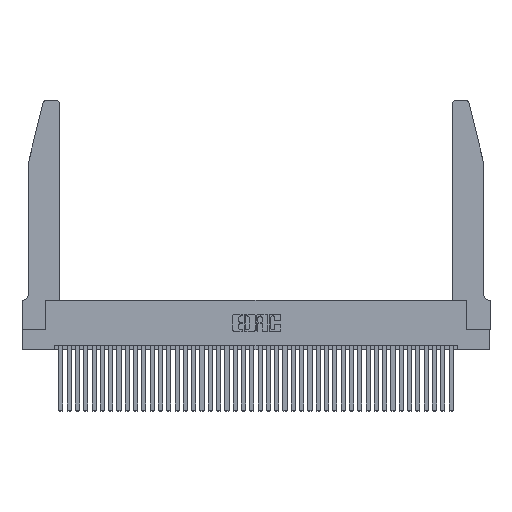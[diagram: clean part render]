
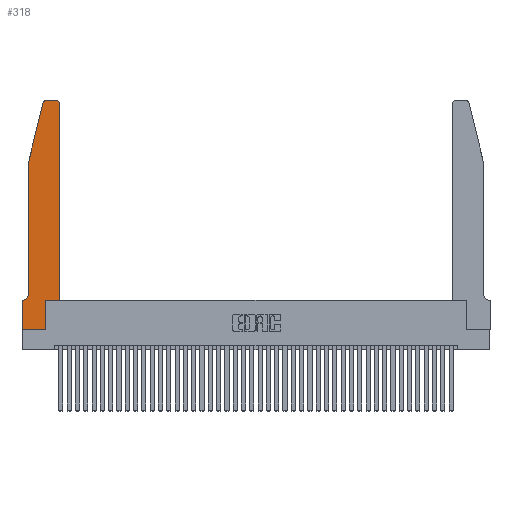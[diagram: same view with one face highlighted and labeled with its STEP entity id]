
A CAD part, top view. The second image highlights one B-rep face of the part: STEP entity #318.
In plain terms, the highlighted planar face has unit normal (0, 0, 1).
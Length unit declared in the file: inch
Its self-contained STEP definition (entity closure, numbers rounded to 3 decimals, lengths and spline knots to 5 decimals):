
#318 = ADVANCED_FACE ( 'NONE', ( #17816 ), #39839, .T. ) ;
#540 = LINE ( 'NONE', #20225, #16574 ) ;
#768 = LINE ( 'NONE', #38268, #39882 ) ;
#1068 = DIRECTION ( 'NONE',  ( 1., 0., 0. ) ) ;
#1900 = EDGE_CURVE ( 'NONE', #9761, #21619, #19135, .T. ) ;
#2062 = VERTEX_POINT ( 'NONE', #34100 ) ;
#3610 = EDGE_CURVE ( 'NONE', #34244, #15719, #6080, .T. ) ;
#3758 = CARTESIAN_POINT ( 'NONE',  ( 0.4505, 0.35, 0.37 ) ) ;
#4036 = EDGE_CURVE ( 'NONE', #32367, #10939, #32556, .T. ) ;
#4038 = DIRECTION ( 'NONE',  ( 1., 0., 0. ) ) ;
#4545 = VECTOR ( 'NONE', #33968, 39.37008 ) ;
#5690 = VECTOR ( 'NONE', #34848, 39.37008 ) ;
#5778 = ORIENTED_EDGE ( 'NONE', *, *, #31699, .T. ) ;
#6080 = LINE ( 'NONE', #30746, #4545 ) ;
#6187 = ORIENTED_EDGE ( 'NONE', *, *, #4036, .T. ) ;
#6251 = EDGE_LOOP ( 'NONE', ( #22858, #30548, #28770, #27454, #10071, #15582, #6848, #36426, #31176, #5778, #37005, #6187 ) ) ;
#6342 = VERTEX_POINT ( 'NONE', #22983 ) ;
#6848 = ORIENTED_EDGE ( 'NONE', *, *, #33665, .T. ) ;
#7501 = CARTESIAN_POINT ( 'NONE',  ( 0.4505, 0.35, 0.37 ) ) ;
#7751 = DIRECTION ( 'NONE',  ( 0., 0., 1. ) ) ;
#8548 = VERTEX_POINT ( 'NONE', #30184 ) ;
#8833 = LINE ( 'NONE', #3758, #40891 ) ;
#9659 = LINE ( 'NONE', #22131, #32171 ) ;
#9676 = LINE ( 'NONE', #38335, #5690 ) ;
#9761 = VERTEX_POINT ( 'NONE', #12002 ) ;
#10027 = DIRECTION ( 'NONE',  ( 0., -1., 0. ) ) ;
#10071 = ORIENTED_EDGE ( 'NONE', *, *, #1900, .T. ) ;
#10304 = DIRECTION ( 'NONE',  ( 0., 0., -1. ) ) ;
#10699 = CIRCLE ( 'NONE', #39131, 0.03 ) ;
#10939 = VERTEX_POINT ( 'NONE', #17354 ) ;
#12002 = CARTESIAN_POINT ( 'NONE',  ( 0.0755, 0.42, 0.37 ) ) ;
#12063 = CARTESIAN_POINT ( 'NONE',  ( 0.284, 2.72, 0.37 ) ) ;
#12916 = EDGE_CURVE ( 'NONE', #40230, #35403, #9676, .T. ) ;
#13436 = LINE ( 'NONE', #16708, #23462 ) ;
#15296 = DIRECTION ( 'NONE',  ( -1., 0., 0. ) ) ;
#15582 = ORIENTED_EDGE ( 'NONE', *, *, #34204, .T. ) ;
#15719 = VERTEX_POINT ( 'NONE', #26855 ) ;
#15876 = EDGE_CURVE ( 'NONE', #15719, #9761, #13436, .T. ) ;
#16203 = CARTESIAN_POINT ( 'NONE',  ( 0.0055, 0.42, 0.37 ) ) ;
#16574 = VECTOR ( 'NONE', #1068, 39.37008 ) ;
#16708 = CARTESIAN_POINT ( 'NONE',  ( 0.0755, 2., 0.37 ) ) ;
#16736 = DIRECTION ( 'NONE',  ( -1., 0., 0. ) ) ;
#17026 = DIRECTION ( 'NONE',  ( 0., 1., 0. ) ) ;
#17354 = CARTESIAN_POINT ( 'NONE',  ( 0.4205, 2.75, 0.37 ) ) ;
#17816 = FACE_OUTER_BOUND ( 'NONE', #6251, .T. ) ;
#17914 = CARTESIAN_POINT ( 'NONE',  ( 0.2865, 0.35, 0.37 ) ) ;
#18338 = DIRECTION ( 'NONE',  ( 0., 0., 1. ) ) ;
#18996 = DIRECTION ( 'NONE',  ( 0., -1., 0. ) ) ;
#19135 = CIRCLE ( 'NONE', #30313, 0.07 ) ;
#19218 = CARTESIAN_POINT ( 'NONE',  ( 0.25487, 2.72718, 0.37 ) ) ;
#20225 = CARTESIAN_POINT ( 'NONE',  ( 0., 0., 0.37 ) ) ;
#21619 = VERTEX_POINT ( 'NONE', #39879 ) ;
#21693 = CARTESIAN_POINT ( 'NONE',  ( 0.2865, 0., 0.37 ) ) ;
#22131 = CARTESIAN_POINT ( 'NONE',  ( 0.2605, 2.75, 0.37 ) ) ;
#22246 = LINE ( 'NONE', #7501, #25759 ) ;
#22758 = CARTESIAN_POINT ( 'NONE',  ( 0., 0., 0.37 ) ) ;
#22858 = ORIENTED_EDGE ( 'NONE', *, *, #36982, .T. ) ;
#22983 = CARTESIAN_POINT ( 'NONE',  ( 0.4505, 0.35, 0.37 ) ) ;
#23462 = VECTOR ( 'NONE', #18996, 39.37008 ) ;
#23572 = DIRECTION ( 'NONE',  ( 1., 0., 0. ) ) ;
#24421 = DIRECTION ( 'NONE',  ( 1., 0., 0. ) ) ;
#25759 = VECTOR ( 'NONE', #17026, 39.37008 ) ;
#25807 = DIRECTION ( 'NONE',  ( -1., 0., 0. ) ) ;
#26855 = CARTESIAN_POINT ( 'NONE',  ( 0.0755, 2., 0.37 ) ) ;
#27083 = AXIS2_PLACEMENT_3D ( 'NONE', #36303, #39684, #32973 ) ;
#27454 = ORIENTED_EDGE ( 'NONE', *, *, #15876, .T. ) ;
#28770 = ORIENTED_EDGE ( 'NONE', *, *, #3610, .T. ) ;
#29844 = CARTESIAN_POINT ( 'NONE',  ( 0.4505, 2.72, 0.37 ) ) ;
#30184 = CARTESIAN_POINT ( 'NONE',  ( 0.284, 2.75, 0.37 ) ) ;
#30313 = AXIS2_PLACEMENT_3D ( 'NONE', #16203, #10304, #16736 ) ;
#30548 = ORIENTED_EDGE ( 'NONE', *, *, #32640, .T. ) ;
#30746 = CARTESIAN_POINT ( 'NONE',  ( 0.0755, 2., 0.37 ) ) ;
#31176 = ORIENTED_EDGE ( 'NONE', *, *, #12916, .T. ) ;
#31699 = EDGE_CURVE ( 'NONE', #35403, #6342, #8833, .T. ) ;
#32171 = VECTOR ( 'NONE', #15296, 39.37008 ) ;
#32367 = VERTEX_POINT ( 'NONE', #29844 ) ;
#32556 = CIRCLE ( 'NONE', #39175, 0.03 ) ;
#32640 = EDGE_CURVE ( 'NONE', #8548, #34244, #10699, .T. ) ;
#32973 = DIRECTION ( 'NONE',  ( 1., 0., 0. ) ) ;
#33665 = EDGE_CURVE ( 'NONE', #2062, #40487, #34979, .T. ) ;
#33968 = DIRECTION ( 'NONE',  ( -0.239, -0.971, 0. ) ) ;
#34100 = CARTESIAN_POINT ( 'NONE',  ( 0., 0.35, 0.37 ) ) ;
#34204 = EDGE_CURVE ( 'NONE', #21619, #2062, #768, .T. ) ;
#34244 = VERTEX_POINT ( 'NONE', #19218 ) ;
#34848 = DIRECTION ( 'NONE',  ( 0., 1., 0. ) ) ;
#34979 = LINE ( 'NONE', #22758, #37505 ) ;
#35403 = VERTEX_POINT ( 'NONE', #17914 ) ;
#35969 = EDGE_CURVE ( 'NONE', #6342, #32367, #22246, .T. ) ;
#35999 = CARTESIAN_POINT ( 'NONE',  ( 0.4205, 2.72, 0.37 ) ) ;
#36303 = CARTESIAN_POINT ( 'NONE',  ( 0., 0.35, 0.37 ) ) ;
#36426 = ORIENTED_EDGE ( 'NONE', *, *, #37821, .T. ) ;
#36982 = EDGE_CURVE ( 'NONE', #10939, #8548, #9659, .T. ) ;
#37005 = ORIENTED_EDGE ( 'NONE', *, *, #35969, .T. ) ;
#37505 = VECTOR ( 'NONE', #10027, 39.37008 ) ;
#37821 = EDGE_CURVE ( 'NONE', #40487, #40230, #540, .T. ) ;
#38268 = CARTESIAN_POINT ( 'NONE',  ( 0.0755, 0.35, 0.37 ) ) ;
#38335 = CARTESIAN_POINT ( 'NONE',  ( 0.2865, 0.35, 0.37 ) ) ;
#39131 = AXIS2_PLACEMENT_3D ( 'NONE', #12063, #18338, #24421 ) ;
#39175 = AXIS2_PLACEMENT_3D ( 'NONE', #35999, #7751, #23572 ) ;
#39597 = CARTESIAN_POINT ( 'NONE',  ( 0., 0., 0.37 ) ) ;
#39684 = DIRECTION ( 'NONE',  ( 0., 0., 1. ) ) ;
#39839 = PLANE ( 'NONE',  #27083 ) ;
#39879 = CARTESIAN_POINT ( 'NONE',  ( 0.0055, 0.35, 0.37 ) ) ;
#39882 = VECTOR ( 'NONE', #25807, 39.37008 ) ;
#40230 = VERTEX_POINT ( 'NONE', #21693 ) ;
#40487 = VERTEX_POINT ( 'NONE', #39597 ) ;
#40891 = VECTOR ( 'NONE', #4038, 39.37008 ) ;
